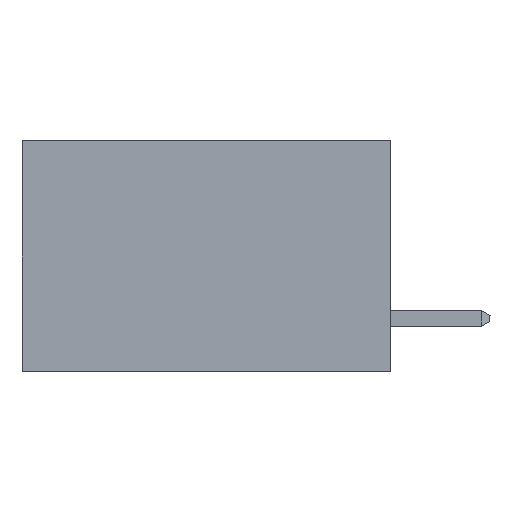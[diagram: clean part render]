
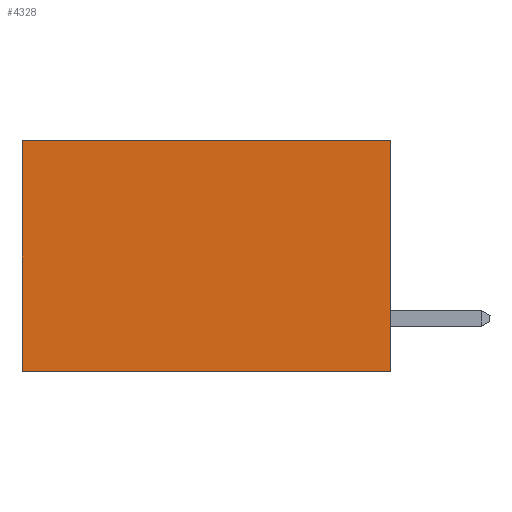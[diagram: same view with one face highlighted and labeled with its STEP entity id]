
A CAD part, left-side view. The second image highlights one B-rep face of the part: STEP entity #4328.
In plain terms, the highlighted planar face has unit normal (-1, 0, 0).
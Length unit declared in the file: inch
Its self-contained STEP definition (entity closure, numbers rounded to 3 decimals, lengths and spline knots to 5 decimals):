
#248 = EDGE_CURVE ( 'NONE', #4817, #8471, #7328, .T. ) ;
#817 = DIRECTION ( 'NONE',  ( 0., 0., -1. ) ) ;
#986 = DIRECTION ( 'NONE',  ( 0., 0., -1. ) ) ;
#1155 = CARTESIAN_POINT ( 'NONE',  ( 0.277, 0., -0.37 ) ) ;
#1478 = CARTESIAN_POINT ( 'NONE',  ( 0.277, 0., -0.37 ) ) ;
#1557 = LINE ( 'NONE', #4419, #9651 ) ;
#1580 = EDGE_LOOP ( 'NONE', ( #4193, #6693, #9042, #2672 ) ) ;
#2039 = EDGE_CURVE ( 'NONE', #4817, #8293, #1557, .T. ) ;
#2083 = DIRECTION ( 'NONE',  ( 0., 1., 0. ) ) ;
#2672 = ORIENTED_EDGE ( 'NONE', *, *, #2039, .T. ) ;
#2700 = EDGE_CURVE ( 'NONE', #8293, #2823, #6038, .T. ) ;
#2823 = VERTEX_POINT ( 'NONE', #7745 ) ;
#3029 = VECTOR ( 'NONE', #9032, 39.37008 ) ;
#3310 = LINE ( 'NONE', #1478, #3029 ) ;
#3365 = CARTESIAN_POINT ( 'NONE',  ( 0.277, 0., 0. ) ) ;
#3672 = DIRECTION ( 'NONE',  ( 1., 0., 0. ) ) ;
#3744 = CARTESIAN_POINT ( 'NONE',  ( 0.277, 0., -0.37 ) ) ;
#3847 = PLANE ( 'NONE',  #9198 ) ;
#4193 = ORIENTED_EDGE ( 'NONE', *, *, #2700, .T. ) ;
#4328 = ADVANCED_FACE ( 'NONE', ( #6007 ), #3847, .F. ) ;
#4419 = CARTESIAN_POINT ( 'NONE',  ( 0.277, 0., 0. ) ) ;
#4817 = VERTEX_POINT ( 'NONE', #3365 ) ;
#4970 = DIRECTION ( 'NONE',  ( 0., 0., -1. ) ) ;
#5167 = VECTOR ( 'NONE', #986, 39.37008 ) ;
#5783 = VECTOR ( 'NONE', #4970, 39.37008 ) ;
#6007 = FACE_OUTER_BOUND ( 'NONE', #1580, .T. ) ;
#6038 = LINE ( 'NONE', #10201, #5783 ) ;
#6651 = CARTESIAN_POINT ( 'NONE',  ( 0.277, 0.59, 0. ) ) ;
#6693 = ORIENTED_EDGE ( 'NONE', *, *, #8297, .F. ) ;
#7328 = LINE ( 'NONE', #3744, #5167 ) ;
#7745 = CARTESIAN_POINT ( 'NONE',  ( 0.277, 0.59, -0.37 ) ) ;
#7944 = CARTESIAN_POINT ( 'NONE',  ( 0.277, 0., -0.37 ) ) ;
#8293 = VERTEX_POINT ( 'NONE', #6651 ) ;
#8297 = EDGE_CURVE ( 'NONE', #8471, #2823, #3310, .T. ) ;
#8471 = VERTEX_POINT ( 'NONE', #7944 ) ;
#9032 = DIRECTION ( 'NONE',  ( 0., 1., 0. ) ) ;
#9042 = ORIENTED_EDGE ( 'NONE', *, *, #248, .F. ) ;
#9198 = AXIS2_PLACEMENT_3D ( 'NONE', #1155, #3672, #817 ) ;
#9651 = VECTOR ( 'NONE', #2083, 39.37008 ) ;
#10201 = CARTESIAN_POINT ( 'NONE',  ( 0.277, 0.59, -0.37 ) ) ;
